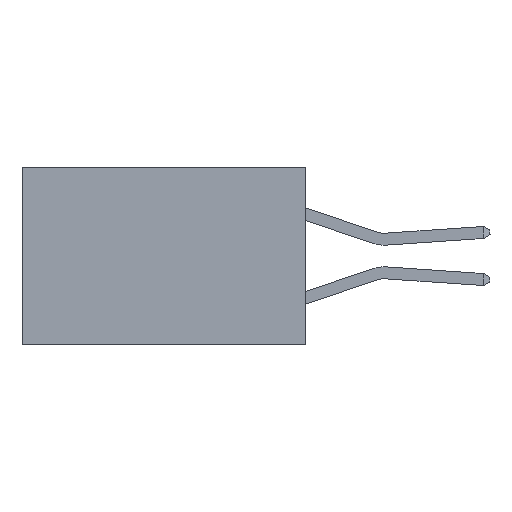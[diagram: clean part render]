
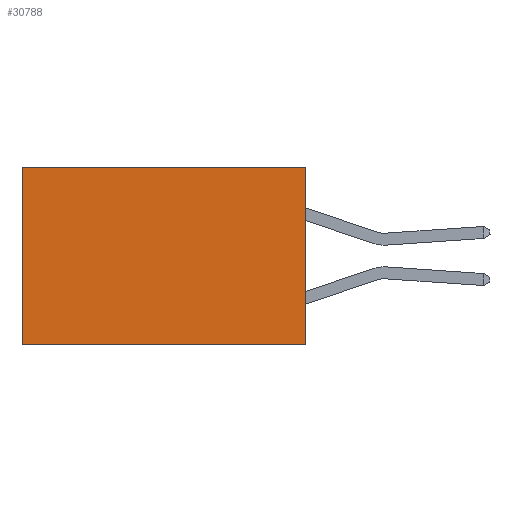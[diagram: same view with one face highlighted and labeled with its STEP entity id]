
A CAD part, left-side view. The second image highlights one B-rep face of the part: STEP entity #30788.
In plain terms, the highlighted planar face has unit normal (-1, 0, 0).
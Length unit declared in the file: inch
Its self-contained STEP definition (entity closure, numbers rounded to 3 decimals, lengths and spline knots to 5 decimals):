
#759 = LINE ( 'NONE', #23334, #12588 ) ;
#2176 = CARTESIAN_POINT ( 'NONE',  ( 0.277, 0., 0. ) ) ;
#2260 = EDGE_CURVE ( 'NONE', #4807, #4656, #759, .T. ) ;
#2878 = DIRECTION ( 'NONE',  ( 0., 0., -1. ) ) ;
#3786 = VECTOR ( 'NONE', #21083, 39.37008 ) ;
#4656 = VERTEX_POINT ( 'NONE', #25459 ) ;
#4807 = VERTEX_POINT ( 'NONE', #2176 ) ;
#5132 = DIRECTION ( 'NONE',  ( 1., 0., 0. ) ) ;
#8462 = CARTESIAN_POINT ( 'NONE',  ( 0.277, 0., 0. ) ) ;
#11248 = EDGE_CURVE ( 'NONE', #13200, #17714, #29464, .T. ) ;
#12588 = VECTOR ( 'NONE', #15996, 39.37008 ) ;
#12726 = ORIENTED_EDGE ( 'NONE', *, *, #18363, .T. ) ;
#13200 = VERTEX_POINT ( 'NONE', #14503 ) ;
#14503 = CARTESIAN_POINT ( 'NONE',  ( 0.277, 0.59, 0. ) ) ;
#14983 = ORIENTED_EDGE ( 'NONE', *, *, #24537, .F. ) ;
#15363 = CARTESIAN_POINT ( 'NONE',  ( 0.277, 0.59, -0.37 ) ) ;
#15996 = DIRECTION ( 'NONE',  ( 0., 0., -1. ) ) ;
#17658 = CARTESIAN_POINT ( 'NONE',  ( 0.277, 0., -0.37 ) ) ;
#17714 = VERTEX_POINT ( 'NONE', #31252 ) ;
#18363 = EDGE_CURVE ( 'NONE', #4807, #13200, #30375, .T. ) ;
#18597 = VECTOR ( 'NONE', #22977, 39.37008 ) ;
#18856 = FACE_OUTER_BOUND ( 'NONE', #28049, .T. ) ;
#19032 = ORIENTED_EDGE ( 'NONE', *, *, #2260, .F. ) ;
#20138 = PLANE ( 'NONE',  #26284 ) ;
#20487 = CARTESIAN_POINT ( 'NONE',  ( 0.277, 0., -0.37 ) ) ;
#21083 = DIRECTION ( 'NONE',  ( 0., 1., 0. ) ) ;
#22056 = VECTOR ( 'NONE', #2878, 39.37008 ) ;
#22187 = ORIENTED_EDGE ( 'NONE', *, *, #11248, .T. ) ;
#22629 = DIRECTION ( 'NONE',  ( 0., 0., -1. ) ) ;
#22977 = DIRECTION ( 'NONE',  ( 0., 1., 0. ) ) ;
#23334 = CARTESIAN_POINT ( 'NONE',  ( 0.277, 0., -0.37 ) ) ;
#24537 = EDGE_CURVE ( 'NONE', #4656, #17714, #31838, .T. ) ;
#25459 = CARTESIAN_POINT ( 'NONE',  ( 0.277, 0., -0.37 ) ) ;
#26284 = AXIS2_PLACEMENT_3D ( 'NONE', #17658, #5132, #22629 ) ;
#28049 = EDGE_LOOP ( 'NONE', ( #22187, #14983, #19032, #12726 ) ) ;
#29464 = LINE ( 'NONE', #15363, #22056 ) ;
#30375 = LINE ( 'NONE', #8462, #3786 ) ;
#30788 = ADVANCED_FACE ( 'NONE', ( #18856 ), #20138, .F. ) ;
#31252 = CARTESIAN_POINT ( 'NONE',  ( 0.277, 0.59, -0.37 ) ) ;
#31838 = LINE ( 'NONE', #20487, #18597 ) ;
